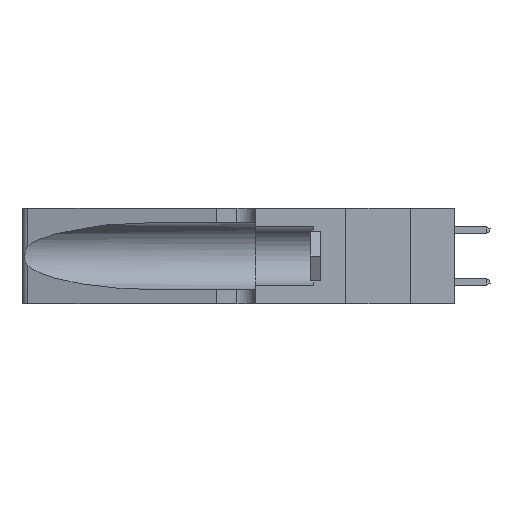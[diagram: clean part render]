
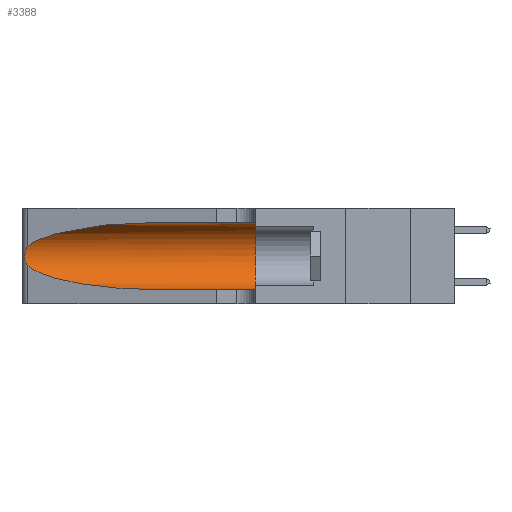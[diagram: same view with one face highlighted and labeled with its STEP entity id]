
A CAD part, left-side view. The second image highlights one B-rep face of the part: STEP entity #3388.
In plain terms, the highlighted cylindrical face has radius 3.308 mm (diameter 6.617 mm), a partial arc.
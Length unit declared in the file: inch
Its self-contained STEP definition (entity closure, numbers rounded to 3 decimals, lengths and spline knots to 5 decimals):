
#312 =( BOUNDED_CURVE ( )  B_SPLINE_CURVE ( 3, ( #24328, #8158, #5758, #10533 ),
 .UNSPECIFIED., .F., .F. ) 
 B_SPLINE_CURVE_WITH_KNOTS ( ( 4, 4 ),
 ( 1.5708, 2.84003 ),
 .UNSPECIFIED. ) 
 CURVE ( )  GEOMETRIC_REPRESENTATION_ITEM ( )  RATIONAL_B_SPLINE_CURVE ( ( 1., 0.87, 0.87, 1. ) ) 
 REPRESENTATION_ITEM ( '' )  );
#729 = CARTESIAN_POINT ( 'NONE',  ( 0.1305, 0.72297, 0.05475 ) ) ;
#959 = B_SPLINE_CURVE_WITH_KNOTS ( 'NONE', 3,
 ( #8702, #11057, #27160, #13335, #29413, #15605, #1641, #17967, #4012, #20310, #6428, #22647, #8809, #24976 ),
 .UNSPECIFIED., .F., .F.,
 ( 4, 2, 2, 2, 2, 2, 4 ),
 ( 0., 0.00027, 0.00053, 0.00107, 0.0016, 0.00187, 0.00214 ),
 .UNSPECIFIED. ) ;
#1641 = CARTESIAN_POINT ( 'NONE',  ( 0.26075, 1.23896, 0.19203 ) ) ;
#1746 = ORIENTED_EDGE ( 'NONE', *, *, #13939, .T. ) ;
#2501 = VERTEX_POINT ( 'NONE', #26700 ) ;
#2906 = VERTEX_POINT ( 'NONE', #25268 ) ;
#3306 = EDGE_CURVE ( 'NONE', #13337, #26549, #312, .T. ) ;
#3388 = ADVANCED_FACE ( 'NONE', ( #22576 ), #15634, .F. ) ;
#3665 = DIRECTION ( 'NONE',  ( 0., 0., -1. ) ) ;
#3867 = EDGE_CURVE ( 'NONE', #2906, #10035, #5404, .T. ) ;
#3934 = EDGE_CURVE ( 'NONE', #10035, #25804, #25077, .T. ) ;
#4012 = CARTESIAN_POINT ( 'NONE',  ( 0.26017, 1.23833, 0.17102 ) ) ;
#4858 = AXIS2_PLACEMENT_3D ( 'NONE', #22765, #8940, #25098 ) ;
#5403 = CARTESIAN_POINT ( 'NONE',  ( 0.25487, 1.22718, 0.14631 ) ) ;
#5404 =( BOUNDED_CURVE ( )  B_SPLINE_CURVE ( 3, ( #5403, #10191, #14766, #729 ),
 .UNSPECIFIED., .F., .F. ) 
 B_SPLINE_CURVE_WITH_KNOTS ( ( 4, 4 ),
 ( 3.44316, 4.71239 ),
 .UNSPECIFIED. ) 
 CURVE ( )  GEOMETRIC_REPRESENTATION_ITEM ( )  RATIONAL_B_SPLINE_CURVE ( ( 1., 0.87, 0.87, 1. ) ) 
 REPRESENTATION_ITEM ( '' )  );
#5758 = CARTESIAN_POINT ( 'NONE',  ( 0.2373, 1.15595, 0.28018 ) ) ;
#6428 = CARTESIAN_POINT ( 'NONE',  ( 0.25789, 1.23486, 0.15765 ) ) ;
#6981 = ORIENTED_EDGE ( 'NONE', *, *, #3867, .T. ) ;
#8120 = CARTESIAN_POINT ( 'NONE',  ( 0.1305, 1.61858, 0.05475 ) ) ;
#8158 = CARTESIAN_POINT ( 'NONE',  ( 0.18966, 0.96281, 0.31525 ) ) ;
#8702 = CARTESIAN_POINT ( 'NONE',  ( 0.25487, 1.22718, 0.22369 ) ) ;
#8809 = CARTESIAN_POINT ( 'NONE',  ( 0.25555, 1.22993, 0.14849 ) ) ;
#8940 = DIRECTION ( 'NONE',  ( 0., 1., 0. ) ) ;
#10035 = VERTEX_POINT ( 'NONE', #12199 ) ;
#10191 = CARTESIAN_POINT ( 'NONE',  ( 0.2373, 1.15595, 0.08982 ) ) ;
#10533 = CARTESIAN_POINT ( 'NONE',  ( 0.25487, 1.22718, 0.22369 ) ) ;
#10807 = CARTESIAN_POINT ( 'NONE',  ( 0.1305, 0.35, 0.05475 ) ) ;
#11057 = CARTESIAN_POINT ( 'NONE',  ( 0.25555, 1.22994, 0.2215 ) ) ;
#12199 = CARTESIAN_POINT ( 'NONE',  ( 0.1305, 0.72297, 0.05475 ) ) ;
#12804 = ORIENTED_EDGE ( 'NONE', *, *, #15729, .F. ) ;
#13097 = DIRECTION ( 'NONE',  ( 0., -1., 0. ) ) ;
#13335 = CARTESIAN_POINT ( 'NONE',  ( 0.25787, 1.23484, 0.2124 ) ) ;
#13337 = VERTEX_POINT ( 'NONE', #25110 ) ;
#13939 = EDGE_CURVE ( 'NONE', #26549, #2906, #959, .T. ) ;
#13983 = AXIS2_PLACEMENT_3D ( 'NONE', #15278, #13097, #3665 ) ;
#14766 = CARTESIAN_POINT ( 'NONE',  ( 0.18966, 0.96281, 0.05475 ) ) ;
#15278 = CARTESIAN_POINT ( 'NONE',  ( 0.1305, 1.61858, 0.185 ) ) ;
#15605 = CARTESIAN_POINT ( 'NONE',  ( 0.26018, 1.23835, 0.19895 ) ) ;
#15634 = CYLINDRICAL_SURFACE ( 'NONE', #13983, 0.13025 ) ;
#15729 = EDGE_CURVE ( 'NONE', #2501, #25804, #26859, .T. ) ;
#16029 = CARTESIAN_POINT ( 'NONE',  ( 0.25487, 1.22718, 0.22369 ) ) ;
#16692 = ORIENTED_EDGE ( 'NONE', *, *, #3306, .T. ) ;
#17369 = DIRECTION ( 'NONE',  ( 0., -1., 0. ) ) ;
#17967 = CARTESIAN_POINT ( 'NONE',  ( 0.26075, 1.23896, 0.178 ) ) ;
#18920 = VECTOR ( 'NONE', #17369, 39.37008 ) ;
#19169 = EDGE_CURVE ( 'NONE', #13337, #2501, #24674, .T. ) ;
#19300 = ORIENTED_EDGE ( 'NONE', *, *, #3934, .T. ) ;
#20310 = CARTESIAN_POINT ( 'NONE',  ( 0.25856, 1.23593, 0.16098 ) ) ;
#22576 = FACE_OUTER_BOUND ( 'NONE', #28834, .T. ) ;
#22647 = CARTESIAN_POINT ( 'NONE',  ( 0.25639, 1.23186, 0.15144 ) ) ;
#22765 = CARTESIAN_POINT ( 'NONE',  ( 0.1305, 0.35, 0.185 ) ) ;
#23453 = DIRECTION ( 'NONE',  ( 0., -1., 0. ) ) ;
#24328 = CARTESIAN_POINT ( 'NONE',  ( 0.1305, 0.72297, 0.31525 ) ) ;
#24674 = LINE ( 'NONE', #28026, #29976 ) ;
#24976 = CARTESIAN_POINT ( 'NONE',  ( 0.25487, 1.22718, 0.14631 ) ) ;
#25077 = LINE ( 'NONE', #8120, #18920 ) ;
#25098 = DIRECTION ( 'NONE',  ( 0., 0., 1. ) ) ;
#25110 = CARTESIAN_POINT ( 'NONE',  ( 0.1305, 0.72297, 0.31525 ) ) ;
#25268 = CARTESIAN_POINT ( 'NONE',  ( 0.25487, 1.22718, 0.14631 ) ) ;
#25804 = VERTEX_POINT ( 'NONE', #10807 ) ;
#25837 = ORIENTED_EDGE ( 'NONE', *, *, #19169, .F. ) ;
#26549 = VERTEX_POINT ( 'NONE', #16029 ) ;
#26700 = CARTESIAN_POINT ( 'NONE',  ( 0.1305, 0.35, 0.31525 ) ) ;
#26859 = CIRCLE ( 'NONE', #4858, 0.13025 ) ;
#27160 = CARTESIAN_POINT ( 'NONE',  ( 0.25639, 1.23184, 0.21858 ) ) ;
#28026 = CARTESIAN_POINT ( 'NONE',  ( 0.1305, 1.61858, 0.31525 ) ) ;
#28834 = EDGE_LOOP ( 'NONE', ( #16692, #1746, #6981, #19300, #12804, #25837 ) ) ;
#29413 = CARTESIAN_POINT ( 'NONE',  ( 0.25854, 1.2359, 0.20912 ) ) ;
#29976 = VECTOR ( 'NONE', #23453, 39.37008 ) ;
